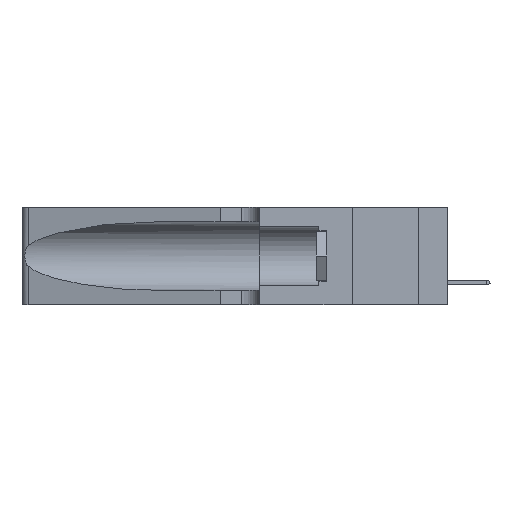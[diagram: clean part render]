
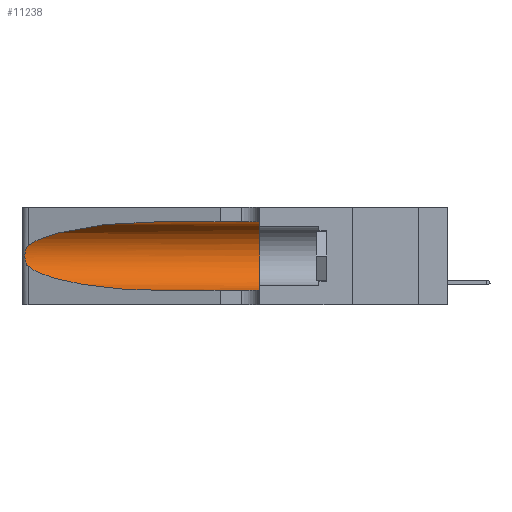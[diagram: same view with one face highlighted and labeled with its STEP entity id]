
A CAD part, left-side view. The second image highlights one B-rep face of the part: STEP entity #11238.
In plain terms, the highlighted cylindrical face has radius 3.308 mm (diameter 6.617 mm), a partial arc.
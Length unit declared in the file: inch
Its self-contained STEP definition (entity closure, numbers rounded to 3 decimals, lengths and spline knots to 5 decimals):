
#58 = CARTESIAN_POINT ( 'NONE',  ( 0.1305, 0.72297, 0.31525 ) ) ;
#105 = CARTESIAN_POINT ( 'NONE',  ( 0.25787, 1.23484, 0.2124 ) ) ;
#219 =( BOUNDED_CURVE ( )  B_SPLINE_CURVE ( 3, ( #27473, #8210, #3446, #27678 ),
 .UNSPECIFIED., .F., .F. ) 
 B_SPLINE_CURVE_WITH_KNOTS ( ( 4, 4 ),
 ( 3.44316, 4.71239 ),
 .UNSPECIFIED. ) 
 CURVE ( )  GEOMETRIC_REPRESENTATION_ITEM ( )  RATIONAL_B_SPLINE_CURVE ( ( 1., 0.87, 0.87, 1. ) ) 
 REPRESENTATION_ITEM ( '' )  );
#2003 = ORIENTED_EDGE ( 'NONE', *, *, #7666, .T. ) ;
#3166 = ORIENTED_EDGE ( 'NONE', *, *, #25903, .F. ) ;
#3446 = CARTESIAN_POINT ( 'NONE',  ( 0.18966, 0.96281, 0.05475 ) ) ;
#4691 = CARTESIAN_POINT ( 'NONE',  ( 0.25487, 1.22718, 0.22369 ) ) ;
#5173 = B_SPLINE_CURVE_WITH_KNOTS ( 'NONE', 3,
 ( #4691, #23958, #12048, #105, #11753, #28515, #21341, #7065, #14056, #23768, #26379, #9444, #28420, #28806 ),
 .UNSPECIFIED., .F., .F.,
 ( 4, 2, 2, 2, 2, 2, 4 ),
 ( 0., 0.00027, 0.00053, 0.00107, 0.0016, 0.00187, 0.00214 ),
 .UNSPECIFIED. ) ;
#5775 =( BOUNDED_CURVE ( )  B_SPLINE_CURVE ( 3, ( #29868, #29980, #8836, #10818 ),
 .UNSPECIFIED., .F., .F. ) 
 B_SPLINE_CURVE_WITH_KNOTS ( ( 4, 4 ),
 ( 1.5708, 2.84003 ),
 .UNSPECIFIED. ) 
 CURVE ( )  GEOMETRIC_REPRESENTATION_ITEM ( )  RATIONAL_B_SPLINE_CURVE ( ( 1., 0.87, 0.87, 1. ) ) 
 REPRESENTATION_ITEM ( '' )  );
#6296 = CARTESIAN_POINT ( 'NONE',  ( 0.1305, 1.61858, 0.05475 ) ) ;
#7065 = CARTESIAN_POINT ( 'NONE',  ( 0.26075, 1.23896, 0.178 ) ) ;
#7666 = EDGE_CURVE ( 'NONE', #15576, #8437, #20920, .T. ) ;
#7923 = CARTESIAN_POINT ( 'NONE',  ( 0.1305, 0.72297, 0.05475 ) ) ;
#8210 = CARTESIAN_POINT ( 'NONE',  ( 0.2373, 1.15595, 0.08982 ) ) ;
#8437 = VERTEX_POINT ( 'NONE', #28979 ) ;
#8524 = VERTEX_POINT ( 'NONE', #24224 ) ;
#8836 = CARTESIAN_POINT ( 'NONE',  ( 0.2373, 1.15595, 0.28018 ) ) ;
#9103 = ORIENTED_EDGE ( 'NONE', *, *, #13021, .T. ) ;
#9444 = CARTESIAN_POINT ( 'NONE',  ( 0.25639, 1.23186, 0.15144 ) ) ;
#10728 = AXIS2_PLACEMENT_3D ( 'NONE', #25532, #20490, #25337 ) ;
#10818 = CARTESIAN_POINT ( 'NONE',  ( 0.25487, 1.22718, 0.22369 ) ) ;
#10884 = DIRECTION ( 'NONE',  ( 0., 0., 1. ) ) ;
#11238 = ADVANCED_FACE ( 'NONE', ( #18442 ), #18113, .F. ) ;
#11304 = DIRECTION ( 'NONE',  ( 0., 1., 0. ) ) ;
#11335 = VERTEX_POINT ( 'NONE', #11402 ) ;
#11402 = CARTESIAN_POINT ( 'NONE',  ( 0.1305, 0.35, 0.31525 ) ) ;
#11536 = AXIS2_PLACEMENT_3D ( 'NONE', #23211, #11304, #10884 ) ;
#11753 = CARTESIAN_POINT ( 'NONE',  ( 0.25854, 1.2359, 0.20912 ) ) ;
#12048 = CARTESIAN_POINT ( 'NONE',  ( 0.25639, 1.23184, 0.21858 ) ) ;
#13021 = EDGE_CURVE ( 'NONE', #30138, #20543, #5775, .T. ) ;
#14056 = CARTESIAN_POINT ( 'NONE',  ( 0.26017, 1.23833, 0.17102 ) ) ;
#14643 = EDGE_CURVE ( 'NONE', #8524, #15576, #219, .T. ) ;
#15576 = VERTEX_POINT ( 'NONE', #7923 ) ;
#18113 = CYLINDRICAL_SURFACE ( 'NONE', #10728, 0.13025 ) ;
#18442 = FACE_OUTER_BOUND ( 'NONE', #23711, .T. ) ;
#18729 = CARTESIAN_POINT ( 'NONE',  ( 0.25487, 1.22718, 0.22369 ) ) ;
#19195 = ORIENTED_EDGE ( 'NONE', *, *, #30845, .T. ) ;
#19232 = LINE ( 'NONE', #25660, #27154 ) ;
#20176 = VECTOR ( 'NONE', #27605, 39.37008 ) ;
#20490 = DIRECTION ( 'NONE',  ( 0., -1., 0. ) ) ;
#20543 = VERTEX_POINT ( 'NONE', #18729 ) ;
#20637 = CIRCLE ( 'NONE', #11536, 0.13025 ) ;
#20920 = LINE ( 'NONE', #6296, #20176 ) ;
#21339 = ORIENTED_EDGE ( 'NONE', *, *, #14643, .T. ) ;
#21341 = CARTESIAN_POINT ( 'NONE',  ( 0.26075, 1.23896, 0.19203 ) ) ;
#23211 = CARTESIAN_POINT ( 'NONE',  ( 0.1305, 0.35, 0.185 ) ) ;
#23711 = EDGE_LOOP ( 'NONE', ( #9103, #19195, #21339, #2003, #24023, #3166 ) ) ;
#23768 = CARTESIAN_POINT ( 'NONE',  ( 0.25856, 1.23593, 0.16098 ) ) ;
#23958 = CARTESIAN_POINT ( 'NONE',  ( 0.25555, 1.22994, 0.2215 ) ) ;
#24023 = ORIENTED_EDGE ( 'NONE', *, *, #27584, .F. ) ;
#24224 = CARTESIAN_POINT ( 'NONE',  ( 0.25487, 1.22718, 0.14631 ) ) ;
#25337 = DIRECTION ( 'NONE',  ( 0., 0., -1. ) ) ;
#25532 = CARTESIAN_POINT ( 'NONE',  ( 0.1305, 1.61858, 0.185 ) ) ;
#25660 = CARTESIAN_POINT ( 'NONE',  ( 0.1305, 1.61858, 0.31525 ) ) ;
#25903 = EDGE_CURVE ( 'NONE', #30138, #11335, #19232, .T. ) ;
#26379 = CARTESIAN_POINT ( 'NONE',  ( 0.25789, 1.23486, 0.15765 ) ) ;
#27154 = VECTOR ( 'NONE', #30176, 39.37008 ) ;
#27473 = CARTESIAN_POINT ( 'NONE',  ( 0.25487, 1.22718, 0.14631 ) ) ;
#27584 = EDGE_CURVE ( 'NONE', #11335, #8437, #20637, .T. ) ;
#27605 = DIRECTION ( 'NONE',  ( 0., -1., 0. ) ) ;
#27678 = CARTESIAN_POINT ( 'NONE',  ( 0.1305, 0.72297, 0.05475 ) ) ;
#28420 = CARTESIAN_POINT ( 'NONE',  ( 0.25555, 1.22993, 0.14849 ) ) ;
#28515 = CARTESIAN_POINT ( 'NONE',  ( 0.26018, 1.23835, 0.19895 ) ) ;
#28806 = CARTESIAN_POINT ( 'NONE',  ( 0.25487, 1.22718, 0.14631 ) ) ;
#28979 = CARTESIAN_POINT ( 'NONE',  ( 0.1305, 0.35, 0.05475 ) ) ;
#29868 = CARTESIAN_POINT ( 'NONE',  ( 0.1305, 0.72297, 0.31525 ) ) ;
#29980 = CARTESIAN_POINT ( 'NONE',  ( 0.18966, 0.96281, 0.31525 ) ) ;
#30138 = VERTEX_POINT ( 'NONE', #58 ) ;
#30176 = DIRECTION ( 'NONE',  ( 0., -1., 0. ) ) ;
#30845 = EDGE_CURVE ( 'NONE', #20543, #8524, #5173, .T. ) ;
